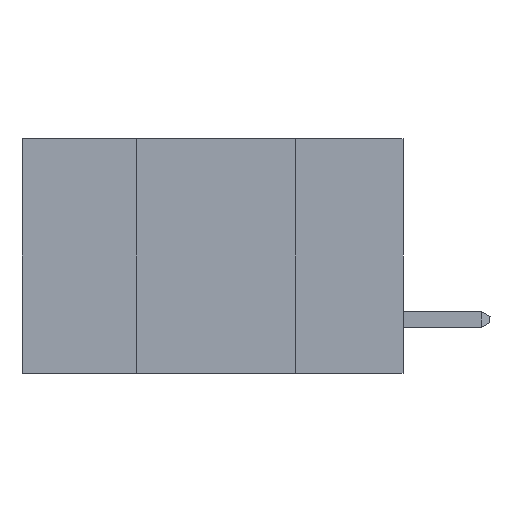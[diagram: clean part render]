
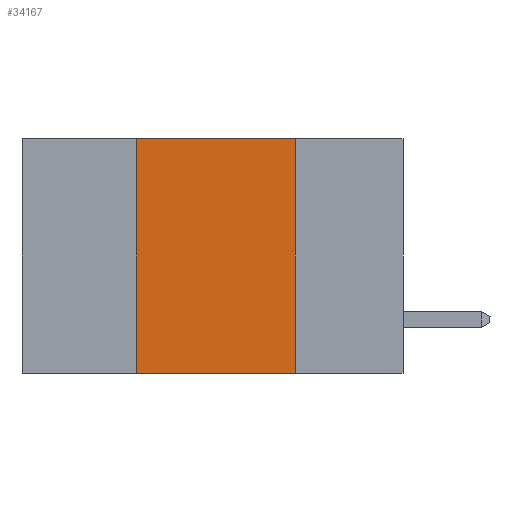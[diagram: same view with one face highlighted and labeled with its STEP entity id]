
A CAD part, left-side view. The second image highlights one B-rep face of the part: STEP entity #34167.
In plain terms, the highlighted planar face has unit normal (-1, 0, 0).
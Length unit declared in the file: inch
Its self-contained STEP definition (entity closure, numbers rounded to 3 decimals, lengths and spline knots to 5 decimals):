
#694 = CARTESIAN_POINT ( 'NONE',  ( 0., 0.6, -0.37 ) ) ;
#1746 = DIRECTION ( 'NONE',  ( 0., 0., 1. ) ) ;
#3408 = EDGE_CURVE ( 'NONE', #32664, #23019, #32276, .T. ) ;
#4562 = CARTESIAN_POINT ( 'NONE',  ( 0., 0.42, 0. ) ) ;
#5217 = DIRECTION ( 'NONE',  ( 0., 0., -1. ) ) ;
#5426 = DIRECTION ( 'NONE',  ( 0., -1., 0. ) ) ;
#5938 = EDGE_LOOP ( 'NONE', ( #12796, #13022, #13200, #18090 ) ) ;
#7850 = CARTESIAN_POINT ( 'NONE',  ( 0., 0.42, -0.37 ) ) ;
#11824 = VECTOR ( 'NONE', #5426, 39.37008 ) ;
#12796 = ORIENTED_EDGE ( 'NONE', *, *, #32692, .F. ) ;
#13022 = ORIENTED_EDGE ( 'NONE', *, *, #26213, .F. ) ;
#13200 = ORIENTED_EDGE ( 'NONE', *, *, #14105, .F. ) ;
#14105 = EDGE_CURVE ( 'NONE', #32664, #36922, #27673, .T. ) ;
#15152 = DIRECTION ( 'NONE',  ( 1., 0., 0. ) ) ;
#17070 = CARTESIAN_POINT ( 'NONE',  ( 0., 0.17, -0.37 ) ) ;
#18090 = ORIENTED_EDGE ( 'NONE', *, *, #3408, .T. ) ;
#19039 = AXIS2_PLACEMENT_3D ( 'NONE', #27186, #15152, #26619 ) ;
#20287 = CARTESIAN_POINT ( 'NONE',  ( 0., 0.17, 0. ) ) ;
#22130 = LINE ( 'NONE', #33602, #30460 ) ;
#22326 = VECTOR ( 'NONE', #1746, 39.37008 ) ;
#23019 = VERTEX_POINT ( 'NONE', #17070 ) ;
#26213 = EDGE_CURVE ( 'NONE', #36922, #35291, #28359, .T. ) ;
#26619 = DIRECTION ( 'NONE',  ( 0., 0., -1. ) ) ;
#26994 = PLANE ( 'NONE',  #19039 ) ;
#27186 = CARTESIAN_POINT ( 'NONE',  ( 0., 0.6, 0. ) ) ;
#27673 = LINE ( 'NONE', #4562, #22326 ) ;
#28359 = LINE ( 'NONE', #31171, #11824 ) ;
#29437 = VECTOR ( 'NONE', #32444, 39.37008 ) ;
#29811 = FACE_OUTER_BOUND ( 'NONE', #5938, .T. ) ;
#30460 = VECTOR ( 'NONE', #5217, 39.37008 ) ;
#31123 = CARTESIAN_POINT ( 'NONE',  ( 0., 0.42, 0. ) ) ;
#31171 = CARTESIAN_POINT ( 'NONE',  ( 0., 0.6, 0. ) ) ;
#32276 = LINE ( 'NONE', #694, #29437 ) ;
#32444 = DIRECTION ( 'NONE',  ( 0., -1., 0. ) ) ;
#32664 = VERTEX_POINT ( 'NONE', #7850 ) ;
#32692 = EDGE_CURVE ( 'NONE', #35291, #23019, #22130, .T. ) ;
#33602 = CARTESIAN_POINT ( 'NONE',  ( 0., 0.17, 0. ) ) ;
#34167 = ADVANCED_FACE ( 'NONE', ( #29811 ), #26994, .F. ) ;
#35291 = VERTEX_POINT ( 'NONE', #20287 ) ;
#36922 = VERTEX_POINT ( 'NONE', #31123 ) ;
